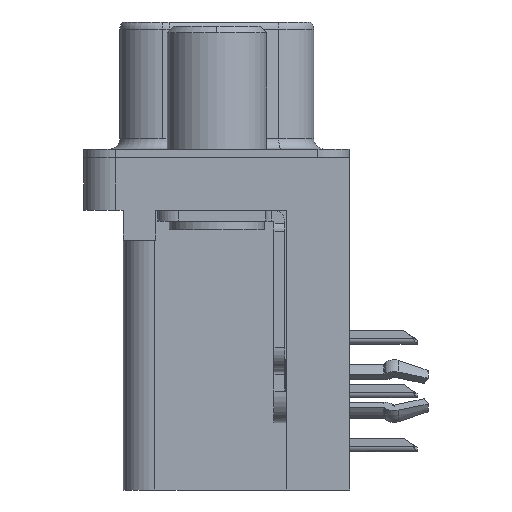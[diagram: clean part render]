
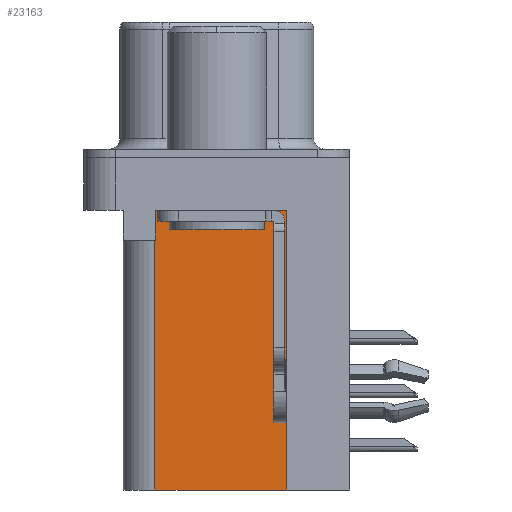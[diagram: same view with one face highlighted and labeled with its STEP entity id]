
A CAD part, left-side view. The second image highlights one B-rep face of the part: STEP entity #23163.
In plain terms, the highlighted planar face has unit normal (-1, 0, 0).
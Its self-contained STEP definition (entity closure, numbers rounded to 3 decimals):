
#126 = VECTOR ( 'NONE', #2833, 1000. ) ;
#443 = CARTESIAN_POINT ( 'NONE',  ( 3.765, -3.295, -15.7 ) ) ;
#448 = LINE ( 'NONE', #2083, #20489 ) ;
#515 = CARTESIAN_POINT ( 'NONE',  ( 3.765, -3.295, -2.5 ) ) ;
#2083 = CARTESIAN_POINT ( 'NONE',  ( 3.765, 2.895, -3.9 ) ) ;
#2704 = DIRECTION ( 'NONE',  ( 0., 0., 1. ) ) ;
#2833 = DIRECTION ( 'NONE',  ( 0., 0., 1. ) ) ;
#3328 = DIRECTION ( 'NONE',  ( 1., 0., 0. ) ) ;
#3354 = VECTOR ( 'NONE', #12726, 1000. ) ;
#3548 = VECTOR ( 'NONE', #7779, 1000. ) ;
#4031 = VECTOR ( 'NONE', #4494, 1000. ) ;
#4494 = DIRECTION ( 'NONE',  ( 0., 1., 0. ) ) ;
#4937 = ORIENTED_EDGE ( 'NONE', *, *, #24550, .F. ) ;
#5754 = EDGE_CURVE ( 'NONE', #9265, #7156, #5876, .T. ) ;
#5876 = LINE ( 'NONE', #6629, #3354 ) ;
#6471 = VERTEX_POINT ( 'NONE', #12717 ) ;
#6629 = CARTESIAN_POINT ( 'NONE',  ( 3.765, -3.295, -2.5 ) ) ;
#7115 = EDGE_CURVE ( 'NONE', #16259, #6471, #8753, .T. ) ;
#7156 = VERTEX_POINT ( 'NONE', #10906 ) ;
#7327 = VERTEX_POINT ( 'NONE', #7375 ) ;
#7375 = CARTESIAN_POINT ( 'NONE',  ( 3.765, 2.895, -3.9 ) ) ;
#7503 = LINE ( 'NONE', #443, #4031 ) ;
#7779 = DIRECTION ( 'NONE',  ( 0., 1., 0. ) ) ;
#7791 = ORIENTED_EDGE ( 'NONE', *, *, #11854, .T. ) ;
#8418 = EDGE_CURVE ( 'NONE', #23245, #9265, #16143, .T. ) ;
#8551 = FACE_OUTER_BOUND ( 'NONE', #20995, .T. ) ;
#8753 = LINE ( 'NONE', #18745, #23994 ) ;
#9265 = VERTEX_POINT ( 'NONE', #515 ) ;
#9735 = AXIS2_PLACEMENT_3D ( 'NONE', #15344, #3328, #17361 ) ;
#10906 = CARTESIAN_POINT ( 'NONE',  ( 3.765, 2.895, -2.5 ) ) ;
#10945 = ORIENTED_EDGE ( 'NONE', *, *, #21380, .T. ) ;
#11854 = EDGE_CURVE ( 'NONE', #7156, #7327, #448, .T. ) ;
#12717 = CARTESIAN_POINT ( 'NONE',  ( 3.765, 2.925, -3.9 ) ) ;
#12726 = DIRECTION ( 'NONE',  ( 0., 1., 0. ) ) ;
#14860 = CARTESIAN_POINT ( 'NONE',  ( 3.765, -3.295, -15.7 ) ) ;
#15344 = CARTESIAN_POINT ( 'NONE',  ( 3.765, -3.295, -15.7 ) ) ;
#15980 = ORIENTED_EDGE ( 'NONE', *, *, #8418, .T. ) ;
#16143 = LINE ( 'NONE', #14860, #126 ) ;
#16259 = VERTEX_POINT ( 'NONE', #16981 ) ;
#16981 = CARTESIAN_POINT ( 'NONE',  ( 3.765, 2.925, -15.7 ) ) ;
#17361 = DIRECTION ( 'NONE',  ( 0., 0., -1. ) ) ;
#18427 = ORIENTED_EDGE ( 'NONE', *, *, #7115, .F. ) ;
#18745 = CARTESIAN_POINT ( 'NONE',  ( 3.765, 2.925, -15.7 ) ) ;
#18904 = LINE ( 'NONE', #19708, #3548 ) ;
#19708 = CARTESIAN_POINT ( 'NONE',  ( 3.765, 0., -3.9 ) ) ;
#20489 = VECTOR ( 'NONE', #24042, 1000. ) ;
#20556 = ORIENTED_EDGE ( 'NONE', *, *, #5754, .T. ) ;
#20995 = EDGE_LOOP ( 'NONE', ( #20556, #7791, #10945, #18427, #4937, #15980 ) ) ;
#21380 = EDGE_CURVE ( 'NONE', #7327, #6471, #18904, .T. ) ;
#23163 = ADVANCED_FACE ( 'NONE', ( #8551 ), #25328, .F. ) ;
#23245 = VERTEX_POINT ( 'NONE', #23513 ) ;
#23513 = CARTESIAN_POINT ( 'NONE',  ( 3.765, -3.295, -15.7 ) ) ;
#23994 = VECTOR ( 'NONE', #2704, 1000. ) ;
#24042 = DIRECTION ( 'NONE',  ( 0., 0., -1. ) ) ;
#24550 = EDGE_CURVE ( 'NONE', #23245, #16259, #7503, .T. ) ;
#25328 = PLANE ( 'NONE',  #9735 ) ;
